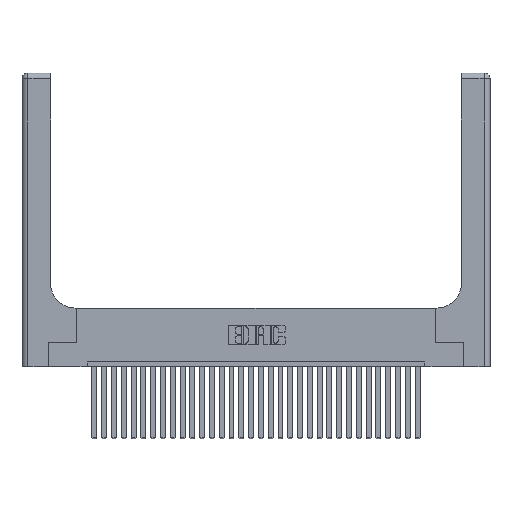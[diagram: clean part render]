
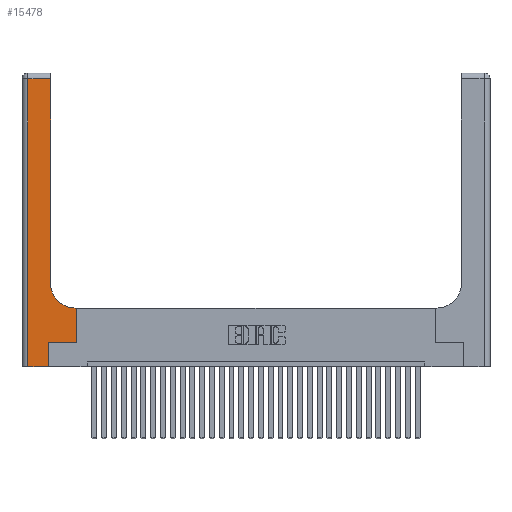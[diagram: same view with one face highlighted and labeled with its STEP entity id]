
A CAD part, top view. The second image highlights one B-rep face of the part: STEP entity #15478.
In plain terms, the highlighted planar face has unit normal (0, 0, 1).
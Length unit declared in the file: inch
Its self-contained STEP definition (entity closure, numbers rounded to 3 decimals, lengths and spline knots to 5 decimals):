
#492 = CARTESIAN_POINT ( 'NONE',  ( 0.5585, 0.6, 0.37 ) ) ;
#1205 = CARTESIAN_POINT ( 'NONE',  ( 0., 3., 0.37 ) ) ;
#1459 = VECTOR ( 'NONE', #25860, 39.37008 ) ;
#2298 = CIRCLE ( 'NONE', #3503, 0.25 ) ;
#2368 = CARTESIAN_POINT ( 'NONE',  ( 0., 0., 0.37 ) ) ;
#3183 = EDGE_CURVE ( 'NONE', #10432, #13941, #2298, .T. ) ;
#3503 = AXIS2_PLACEMENT_3D ( 'NONE', #16167, #23627, #21405 ) ;
#3670 = ORIENTED_EDGE ( 'NONE', *, *, #3183, .T. ) ;
#4106 = LINE ( 'NONE', #15916, #1459 ) ;
#4506 = DIRECTION ( 'NONE',  ( 1., 0., 0. ) ) ;
#4574 = EDGE_CURVE ( 'NONE', #12631, #10432, #13599, .T. ) ;
#5712 = DIRECTION ( 'NONE',  ( 0., 1., 0. ) ) ;
#6405 = VECTOR ( 'NONE', #15942, 39.37008 ) ;
#6409 = EDGE_CURVE ( 'NONE', #19045, #10233, #21832, .T. ) ;
#6830 = CARTESIAN_POINT ( 'NONE',  ( 0.5415, 0.6, 0.37 ) ) ;
#7108 = LINE ( 'NONE', #24312, #25447 ) ;
#8334 = LINE ( 'NONE', #22598, #6405 ) ;
#8622 = EDGE_CURVE ( 'NONE', #23779, #22524, #4106, .T. ) ;
#8632 = LINE ( 'NONE', #2368, #23142 ) ;
#9176 = CARTESIAN_POINT ( 'NONE',  ( 0.06, 0., 0.37 ) ) ;
#10128 = CARTESIAN_POINT ( 'NONE',  ( 0.2915, 2.94, 0.37 ) ) ;
#10233 = VERTEX_POINT ( 'NONE', #28196 ) ;
#10269 = AXIS2_PLACEMENT_3D ( 'NONE', #1205, #20710, #18560 ) ;
#10432 = VERTEX_POINT ( 'NONE', #6830 ) ;
#12146 = CARTESIAN_POINT ( 'NONE',  ( 0.269, 0., 0.37 ) ) ;
#12293 = VERTEX_POINT ( 'NONE', #10128 ) ;
#12439 = VERTEX_POINT ( 'NONE', #21921 ) ;
#12631 = VERTEX_POINT ( 'NONE', #492 ) ;
#12774 = EDGE_CURVE ( 'NONE', #13941, #12293, #22875, .T. ) ;
#13086 = ORIENTED_EDGE ( 'NONE', *, *, #14513, .T. ) ;
#13556 = EDGE_CURVE ( 'NONE', #12439, #12631, #8334, .T. ) ;
#13599 = LINE ( 'NONE', #25724, #20883 ) ;
#13941 = VERTEX_POINT ( 'NONE', #16394 ) ;
#14059 = ORIENTED_EDGE ( 'NONE', *, *, #6409, .T. ) ;
#14513 = EDGE_CURVE ( 'NONE', #22524, #19045, #8632, .T. ) ;
#14602 = DIRECTION ( 'NONE',  ( 1., 0., 0. ) ) ;
#14693 = ORIENTED_EDGE ( 'NONE', *, *, #8622, .T. ) ;
#15478 = ADVANCED_FACE ( 'NONE', ( #20820 ), #28008, .F. ) ;
#15605 = CARTESIAN_POINT ( 'NONE',  ( 0.2915, 3., 0.37 ) ) ;
#15916 = CARTESIAN_POINT ( 'NONE',  ( 0.06, 3., 0.37 ) ) ;
#15942 = DIRECTION ( 'NONE',  ( 0., 1., 0. ) ) ;
#15963 = ORIENTED_EDGE ( 'NONE', *, *, #31675, .T. ) ;
#16167 = CARTESIAN_POINT ( 'NONE',  ( 0.5415, 0.85, 0.37 ) ) ;
#16394 = CARTESIAN_POINT ( 'NONE',  ( 0.2915, 0.85, 0.37 ) ) ;
#18363 = VECTOR ( 'NONE', #22108, 39.37008 ) ;
#18560 = DIRECTION ( 'NONE',  ( -1., 0., 0. ) ) ;
#18770 = CARTESIAN_POINT ( 'NONE',  ( 0.269, 0.25, 0.37 ) ) ;
#19045 = VERTEX_POINT ( 'NONE', #31449 ) ;
#19256 = DIRECTION ( 'NONE',  ( -1., 0., 0. ) ) ;
#19795 = VECTOR ( 'NONE', #5712, 39.37008 ) ;
#20596 = ORIENTED_EDGE ( 'NONE', *, *, #21166, .T. ) ;
#20710 = DIRECTION ( 'NONE',  ( 0., 0., -1. ) ) ;
#20820 = FACE_OUTER_BOUND ( 'NONE', #24213, .T. ) ;
#20883 = VECTOR ( 'NONE', #30377, 39.37008 ) ;
#21166 = EDGE_CURVE ( 'NONE', #12293, #23779, #7108, .T. ) ;
#21400 = VECTOR ( 'NONE', #4506, 39.37008 ) ;
#21405 = DIRECTION ( 'NONE',  ( 1., 0., 0. ) ) ;
#21814 = ORIENTED_EDGE ( 'NONE', *, *, #4574, .T. ) ;
#21832 = LINE ( 'NONE', #12146, #18363 ) ;
#21921 = CARTESIAN_POINT ( 'NONE',  ( 0.5585, 0.25, 0.37 ) ) ;
#22108 = DIRECTION ( 'NONE',  ( 0., 1., 0. ) ) ;
#22524 = VERTEX_POINT ( 'NONE', #9176 ) ;
#22598 = CARTESIAN_POINT ( 'NONE',  ( 0.5585, 0.25, 0.37 ) ) ;
#22875 = LINE ( 'NONE', #15605, #19795 ) ;
#23142 = VECTOR ( 'NONE', #14602, 39.37008 ) ;
#23627 = DIRECTION ( 'NONE',  ( 0., 0., -1. ) ) ;
#23779 = VERTEX_POINT ( 'NONE', #29220 ) ;
#24213 = EDGE_LOOP ( 'NONE', ( #30574, #20596, #14693, #13086, #14059, #15963, #25367, #21814, #3670 ) ) ;
#24312 = CARTESIAN_POINT ( 'NONE',  ( 0., 2.94, 0.37 ) ) ;
#25367 = ORIENTED_EDGE ( 'NONE', *, *, #13556, .T. ) ;
#25447 = VECTOR ( 'NONE', #19256, 39.37008 ) ;
#25724 = CARTESIAN_POINT ( 'NONE',  ( 0.2915, 0.6, 0.37 ) ) ;
#25860 = DIRECTION ( 'NONE',  ( 0., -1., 0. ) ) ;
#28008 = PLANE ( 'NONE',  #10269 ) ;
#28196 = CARTESIAN_POINT ( 'NONE',  ( 0.269, 0.25, 0.37 ) ) ;
#28708 = LINE ( 'NONE', #18770, #21400 ) ;
#29220 = CARTESIAN_POINT ( 'NONE',  ( 0.06, 2.94, 0.37 ) ) ;
#30377 = DIRECTION ( 'NONE',  ( -1., 0., 0. ) ) ;
#30574 = ORIENTED_EDGE ( 'NONE', *, *, #12774, .T. ) ;
#31449 = CARTESIAN_POINT ( 'NONE',  ( 0.269, 0., 0.37 ) ) ;
#31675 = EDGE_CURVE ( 'NONE', #10233, #12439, #28708, .T. ) ;
